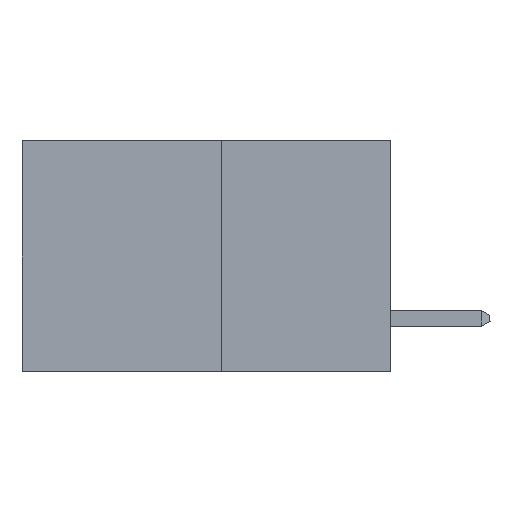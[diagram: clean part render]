
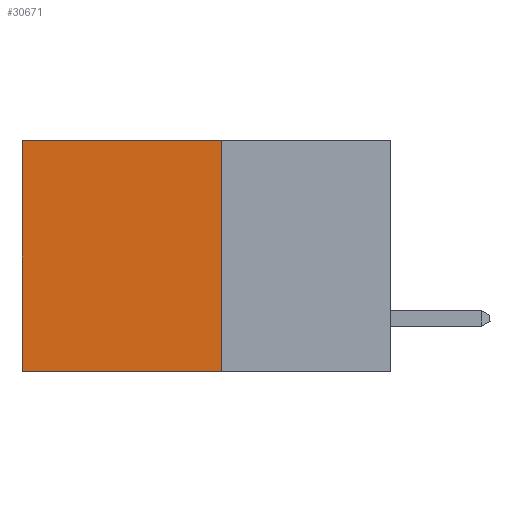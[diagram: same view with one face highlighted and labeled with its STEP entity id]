
A CAD part, left-side view. The second image highlights one B-rep face of the part: STEP entity #30671.
In plain terms, the highlighted planar face has unit normal (-1, 0, 0).
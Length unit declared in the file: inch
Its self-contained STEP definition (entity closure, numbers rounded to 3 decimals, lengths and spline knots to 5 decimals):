
#435 = ORIENTED_EDGE ( 'NONE', *, *, #25527, .F. ) ;
#2836 = DIRECTION ( 'NONE',  ( 0., 1., 0. ) ) ;
#2874 = VERTEX_POINT ( 'NONE', #31179 ) ;
#4195 = ORIENTED_EDGE ( 'NONE', *, *, #10296, .T. ) ;
#5730 = DIRECTION ( 'NONE',  ( 1., 0., 0. ) ) ;
#5910 = DIRECTION ( 'NONE',  ( 0., 1., 0. ) ) ;
#6141 = VERTEX_POINT ( 'NONE', #19684 ) ;
#6241 = PLANE ( 'NONE',  #16727 ) ;
#8006 = VERTEX_POINT ( 'NONE', #27188 ) ;
#8861 = FACE_OUTER_BOUND ( 'NONE', #14420, .T. ) ;
#9769 = LINE ( 'NONE', #24319, #29877 ) ;
#9938 = VECTOR ( 'NONE', #25611, 39.37008 ) ;
#10296 = EDGE_CURVE ( 'NONE', #2874, #6141, #9769, .T. ) ;
#10680 = CARTESIAN_POINT ( 'NONE',  ( 0.277, 0.27, -0.37 ) ) ;
#11047 = CARTESIAN_POINT ( 'NONE',  ( 0.277, 0.59, -0.37 ) ) ;
#13129 = CARTESIAN_POINT ( 'NONE',  ( 0.277, 0.27, -0.37 ) ) ;
#14420 = EDGE_LOOP ( 'NONE', ( #33213, #19188, #435, #4195 ) ) ;
#16727 = AXIS2_PLACEMENT_3D ( 'NONE', #21489, #5730, #24138 ) ;
#19188 = ORIENTED_EDGE ( 'NONE', *, *, #22883, .F. ) ;
#19271 = LINE ( 'NONE', #10680, #25423 ) ;
#19381 = LINE ( 'NONE', #30755, #9938 ) ;
#19684 = CARTESIAN_POINT ( 'NONE',  ( 0.277, 0.59, 0. ) ) ;
#21489 = CARTESIAN_POINT ( 'NONE',  ( 0.277, 0.27, -0.37 ) ) ;
#22298 = VERTEX_POINT ( 'NONE', #11047 ) ;
#22883 = EDGE_CURVE ( 'NONE', #8006, #22298, #19271, .T. ) ;
#24138 = DIRECTION ( 'NONE',  ( 0., 0., -1. ) ) ;
#24319 = CARTESIAN_POINT ( 'NONE',  ( 0.277, 0.27, 0. ) ) ;
#25423 = VECTOR ( 'NONE', #2836, 39.37008 ) ;
#25527 = EDGE_CURVE ( 'NONE', #2874, #8006, #28257, .T. ) ;
#25611 = DIRECTION ( 'NONE',  ( 0., 0., -1. ) ) ;
#27188 = CARTESIAN_POINT ( 'NONE',  ( 0.277, 0.27, -0.37 ) ) ;
#28257 = LINE ( 'NONE', #13129, #29907 ) ;
#29877 = VECTOR ( 'NONE', #5910, 39.37008 ) ;
#29907 = VECTOR ( 'NONE', #31471, 39.37008 ) ;
#30671 = ADVANCED_FACE ( 'NONE', ( #8861 ), #6241, .F. ) ;
#30755 = CARTESIAN_POINT ( 'NONE',  ( 0.277, 0.59, -0.37 ) ) ;
#31179 = CARTESIAN_POINT ( 'NONE',  ( 0.277, 0.27, 0. ) ) ;
#31471 = DIRECTION ( 'NONE',  ( 0., 0., -1. ) ) ;
#32902 = EDGE_CURVE ( 'NONE', #6141, #22298, #19381, .T. ) ;
#33213 = ORIENTED_EDGE ( 'NONE', *, *, #32902, .T. ) ;
